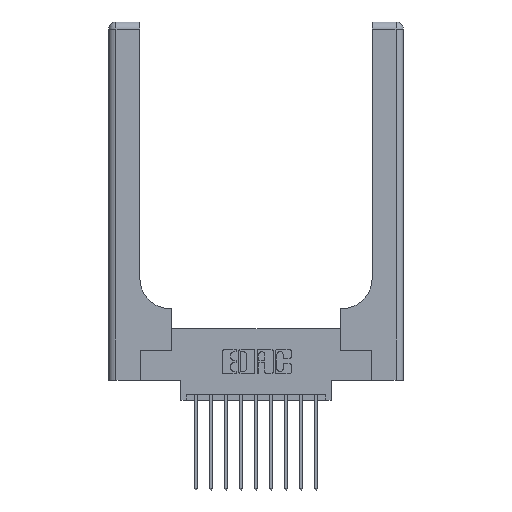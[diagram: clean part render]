
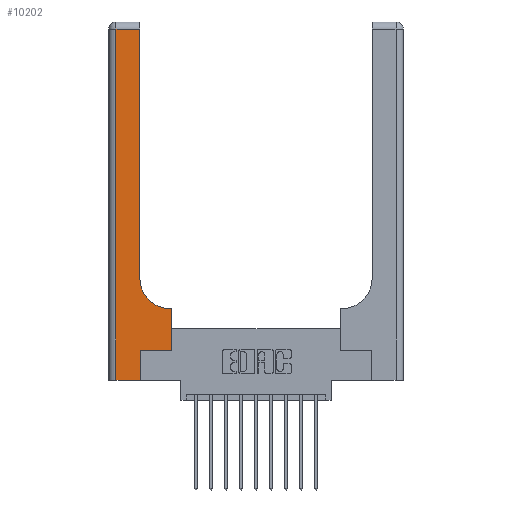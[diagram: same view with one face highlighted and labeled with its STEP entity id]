
A CAD part, top view. The second image highlights one B-rep face of the part: STEP entity #10202.
In plain terms, the highlighted planar face has unit normal (0, 0, 1).
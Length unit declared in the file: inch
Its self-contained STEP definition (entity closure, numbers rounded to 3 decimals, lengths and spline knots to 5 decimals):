
#21 = AXIS2_PLACEMENT_3D ( 'NONE', #6627, #14995, #7834 ) ;
#143 = VECTOR ( 'NONE', #866, 39.37008 ) ;
#180 = VERTEX_POINT ( 'NONE', #2380 ) ;
#302 = LINE ( 'NONE', #9665, #6449 ) ;
#521 = VERTEX_POINT ( 'NONE', #2989 ) ;
#713 = ORIENTED_EDGE ( 'NONE', *, *, #2098, .T. ) ;
#730 = VERTEX_POINT ( 'NONE', #5438 ) ;
#828 = VERTEX_POINT ( 'NONE', #2919 ) ;
#837 = CARTESIAN_POINT ( 'NONE',  ( 0.528, 0.6, 0.37 ) ) ;
#866 = DIRECTION ( 'NONE',  ( -1., 0., 0. ) ) ;
#898 = CARTESIAN_POINT ( 'NONE',  ( 0., 2.94, 0.37 ) ) ;
#1107 = CIRCLE ( 'NONE', #21, 0.25 ) ;
#1282 = VERTEX_POINT ( 'NONE', #9304 ) ;
#1476 = CARTESIAN_POINT ( 'NONE',  ( 0.265, 0.25, 0.37 ) ) ;
#1646 = DIRECTION ( 'NONE',  ( 0., 1., 0. ) ) ;
#1703 = VERTEX_POINT ( 'NONE', #4764 ) ;
#2098 = EDGE_CURVE ( 'NONE', #730, #1282, #12673, .T. ) ;
#2267 = EDGE_CURVE ( 'NONE', #2504, #1703, #1107, .T. ) ;
#2380 = CARTESIAN_POINT ( 'NONE',  ( 0.06, 0., 0.37 ) ) ;
#2504 = VERTEX_POINT ( 'NONE', #11810 ) ;
#2919 = CARTESIAN_POINT ( 'NONE',  ( 0.528, 0.25, 0.37 ) ) ;
#2925 = CARTESIAN_POINT ( 'NONE',  ( 0., 3., 0.37 ) ) ;
#2989 = CARTESIAN_POINT ( 'NONE',  ( 0.265, 0., 0.37 ) ) ;
#3134 = LINE ( 'NONE', #12583, #9603 ) ;
#3596 = DIRECTION ( 'NONE',  ( -1., 0., 0. ) ) ;
#3669 = VECTOR ( 'NONE', #14755, 39.37008 ) ;
#4079 = ORIENTED_EDGE ( 'NONE', *, *, #2267, .T. ) ;
#4695 = ORIENTED_EDGE ( 'NONE', *, *, #14625, .T. ) ;
#4764 = CARTESIAN_POINT ( 'NONE',  ( 0.26, 0.85, 0.37 ) ) ;
#4795 = ORIENTED_EDGE ( 'NONE', *, *, #5600, .T. ) ;
#5008 = CARTESIAN_POINT ( 'NONE',  ( 0.265, 0.25, 0.37 ) ) ;
#5203 = VECTOR ( 'NONE', #12277, 39.37008 ) ;
#5381 = DIRECTION ( 'NONE',  ( 0., 1., 0. ) ) ;
#5438 = CARTESIAN_POINT ( 'NONE',  ( 0.26, 2.94, 0.37 ) ) ;
#5600 = EDGE_CURVE ( 'NONE', #521, #10546, #8804, .T. ) ;
#5798 = DIRECTION ( 'NONE',  ( 1., 0., 0. ) ) ;
#6449 = VECTOR ( 'NONE', #3596, 39.37008 ) ;
#6627 = CARTESIAN_POINT ( 'NONE',  ( 0.51, 0.85, 0.37 ) ) ;
#6637 = DIRECTION ( 'NONE',  ( 0., 0., -1. ) ) ;
#6851 = CARTESIAN_POINT ( 'NONE',  ( 0.06, 3., 0.37 ) ) ;
#6962 = VECTOR ( 'NONE', #1646, 39.37008 ) ;
#6968 = CARTESIAN_POINT ( 'NONE',  ( 0., 0., 0.37 ) ) ;
#7304 = LINE ( 'NONE', #1476, #3669 ) ;
#7834 = DIRECTION ( 'NONE',  ( 1., 0., 0. ) ) ;
#8267 = VECTOR ( 'NONE', #5798, 39.37008 ) ;
#8653 = CARTESIAN_POINT ( 'NONE',  ( 0.265, 0., 0.37 ) ) ;
#8677 = ORIENTED_EDGE ( 'NONE', *, *, #9268, .T. ) ;
#8804 = LINE ( 'NONE', #8653, #5203 ) ;
#9268 = EDGE_CURVE ( 'NONE', #15256, #2504, #302, .T. ) ;
#9304 = CARTESIAN_POINT ( 'NONE',  ( 0.06, 2.94, 0.37 ) ) ;
#9384 = AXIS2_PLACEMENT_3D ( 'NONE', #2925, #6637, #15007 ) ;
#9603 = VECTOR ( 'NONE', #5381, 39.37008 ) ;
#9620 = FACE_OUTER_BOUND ( 'NONE', #13904, .T. ) ;
#9665 = CARTESIAN_POINT ( 'NONE',  ( 0.26, 0.6, 0.37 ) ) ;
#10202 = ADVANCED_FACE ( 'NONE', ( #9620 ), #10203, .F. ) ;
#10203 = PLANE ( 'NONE',  #9384 ) ;
#10312 = VECTOR ( 'NONE', #12874, 39.37008 ) ;
#10546 = VERTEX_POINT ( 'NONE', #5008 ) ;
#10680 = EDGE_CURVE ( 'NONE', #828, #15256, #3134, .T. ) ;
#10879 = ORIENTED_EDGE ( 'NONE', *, *, #13233, .T. ) ;
#11073 = ORIENTED_EDGE ( 'NONE', *, *, #10680, .T. ) ;
#11810 = CARTESIAN_POINT ( 'NONE',  ( 0.51, 0.6, 0.37 ) ) ;
#12277 = DIRECTION ( 'NONE',  ( 0., 1., 0. ) ) ;
#12459 = CARTESIAN_POINT ( 'NONE',  ( 0.26, 3., 0.37 ) ) ;
#12583 = CARTESIAN_POINT ( 'NONE',  ( 0.528, 0.25, 0.37 ) ) ;
#12673 = LINE ( 'NONE', #898, #143 ) ;
#12721 = ORIENTED_EDGE ( 'NONE', *, *, #15210, .T. ) ;
#12730 = ORIENTED_EDGE ( 'NONE', *, *, #14968, .T. ) ;
#12874 = DIRECTION ( 'NONE',  ( 0., -1., 0. ) ) ;
#13233 = EDGE_CURVE ( 'NONE', #1703, #730, #13330, .T. ) ;
#13330 = LINE ( 'NONE', #12459, #6962 ) ;
#13471 = LINE ( 'NONE', #6851, #10312 ) ;
#13904 = EDGE_LOOP ( 'NONE', ( #10879, #713, #12721, #4695, #4795, #12730, #11073, #8677, #4079 ) ) ;
#14621 = LINE ( 'NONE', #6968, #8267 ) ;
#14625 = EDGE_CURVE ( 'NONE', #180, #521, #14621, .T. ) ;
#14755 = DIRECTION ( 'NONE',  ( 1., 0., 0. ) ) ;
#14968 = EDGE_CURVE ( 'NONE', #10546, #828, #7304, .T. ) ;
#14995 = DIRECTION ( 'NONE',  ( 0., 0., -1. ) ) ;
#15007 = DIRECTION ( 'NONE',  ( -1., 0., 0. ) ) ;
#15210 = EDGE_CURVE ( 'NONE', #1282, #180, #13471, .T. ) ;
#15256 = VERTEX_POINT ( 'NONE', #837 ) ;
